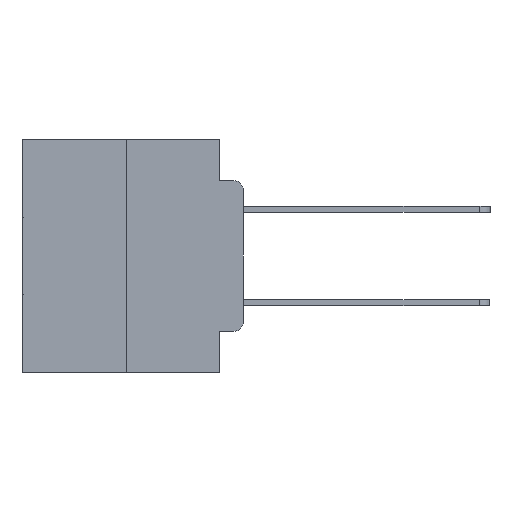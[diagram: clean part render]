
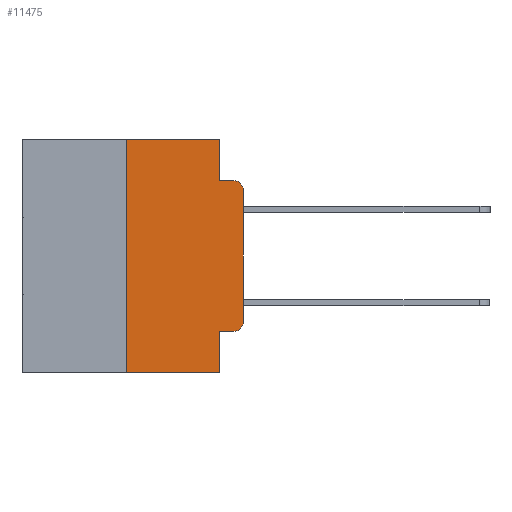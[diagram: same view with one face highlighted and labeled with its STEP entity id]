
A CAD part, left-side view. The second image highlights one B-rep face of the part: STEP entity #11475.
In plain terms, the highlighted planar face has unit normal (-1, 0, 0).
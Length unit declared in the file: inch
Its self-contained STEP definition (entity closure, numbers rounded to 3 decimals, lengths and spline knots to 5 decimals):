
#230 = ORIENTED_EDGE ( 'NONE', *, *, #17750, .T. ) ;
#252 = LINE ( 'NONE', #5214, #23738 ) ;
#612 = ORIENTED_EDGE ( 'NONE', *, *, #15065, .T. ) ;
#625 = EDGE_CURVE ( 'NONE', #12171, #2287, #17639, .T. ) ;
#962 = ORIENTED_EDGE ( 'NONE', *, *, #28681, .F. ) ;
#1080 = VERTEX_POINT ( 'NONE', #4352 ) ;
#1365 = LINE ( 'NONE', #23403, #6791 ) ;
#1390 = FACE_OUTER_BOUND ( 'NONE', #8473, .T. ) ;
#1989 = DIRECTION ( 'NONE',  ( 0., -1., 0. ) ) ;
#2067 = DIRECTION ( 'NONE',  ( -1., 0., 0. ) ) ;
#2287 = VERTEX_POINT ( 'NONE', #5164 ) ;
#2315 = CIRCLE ( 'NONE', #28119, 0.02 ) ;
#3079 = DIRECTION ( 'NONE',  ( -1., 0., 0. ) ) ;
#3886 = ORIENTED_EDGE ( 'NONE', *, *, #11709, .F. ) ;
#4024 = EDGE_CURVE ( 'NONE', #12171, #8507, #252, .T. ) ;
#4352 = CARTESIAN_POINT ( 'NONE',  ( 0., 0.051, 0. ) ) ;
#4429 = CARTESIAN_POINT ( 'NONE',  ( 0., 0.25, 0. ) ) ;
#4977 = LINE ( 'NONE', #8878, #28189 ) ;
#5164 = CARTESIAN_POINT ( 'NONE',  ( 0., 0.051, -0.5 ) ) ;
#5214 = CARTESIAN_POINT ( 'NONE',  ( 0., 0.25, 0. ) ) ;
#5328 = CARTESIAN_POINT ( 'NONE',  ( 0., 0.473, -0.5 ) ) ;
#5348 = CARTESIAN_POINT ( 'NONE',  ( 0., 0., -0.1085 ) ) ;
#5417 = CARTESIAN_POINT ( 'NONE',  ( 0., 0.473, 0. ) ) ;
#5999 = DIRECTION ( 'NONE',  ( 0., -1., 0. ) ) ;
#6517 = EDGE_CURVE ( 'NONE', #9970, #18839, #2315, .T. ) ;
#6551 = VERTEX_POINT ( 'NONE', #18151 ) ;
#6791 = VECTOR ( 'NONE', #10105, 39.37008 ) ;
#6991 = LINE ( 'NONE', #15719, #7715 ) ;
#7275 = VERTEX_POINT ( 'NONE', #16354 ) ;
#7715 = VECTOR ( 'NONE', #1989, 39.37008 ) ;
#7823 = ORIENTED_EDGE ( 'NONE', *, *, #12040, .F. ) ;
#8458 = EDGE_CURVE ( 'NONE', #6551, #18839, #6991, .T. ) ;
#8473 = EDGE_LOOP ( 'NONE', ( #230, #12473, #25096, #962, #7823, #20603, #8550, #3886, #21295, #612 ) ) ;
#8507 = VERTEX_POINT ( 'NONE', #4429 ) ;
#8550 = ORIENTED_EDGE ( 'NONE', *, *, #625, .T. ) ;
#8878 = CARTESIAN_POINT ( 'NONE',  ( 0., 0.473, 0. ) ) ;
#8984 = EDGE_CURVE ( 'NONE', #25645, #19336, #23582, .T. ) ;
#9636 = CIRCLE ( 'NONE', #21478, 0.02 ) ;
#9970 = VERTEX_POINT ( 'NONE', #5348 ) ;
#10105 = DIRECTION ( 'NONE',  ( 0., 0., -1. ) ) ;
#11475 = ADVANCED_FACE ( 'NONE', ( #1390 ), #21213, .F. ) ;
#11626 = VECTOR ( 'NONE', #5999, 39.37008 ) ;
#11639 = VECTOR ( 'NONE', #16133, 39.37008 ) ;
#11709 = EDGE_CURVE ( 'NONE', #25645, #2287, #1365, .T. ) ;
#12040 = EDGE_CURVE ( 'NONE', #8507, #1080, #4977, .T. ) ;
#12086 = DIRECTION ( 'NONE',  ( 0., 0., 1. ) ) ;
#12171 = VERTEX_POINT ( 'NONE', #13817 ) ;
#12231 = CARTESIAN_POINT ( 'NONE',  ( 0., 0.02, -0.0885 ) ) ;
#12473 = ORIENTED_EDGE ( 'NONE', *, *, #6517, .T. ) ;
#13605 = AXIS2_PLACEMENT_3D ( 'NONE', #5417, #27938, #14601 ) ;
#13817 = CARTESIAN_POINT ( 'NONE',  ( 0., 0.25, -0.5 ) ) ;
#14601 = DIRECTION ( 'NONE',  ( 0., 0., -1. ) ) ;
#15065 = EDGE_CURVE ( 'NONE', #19336, #7275, #9636, .T. ) ;
#15082 = CARTESIAN_POINT ( 'NONE',  ( 0., 0.051, -0.4115 ) ) ;
#15719 = CARTESIAN_POINT ( 'NONE',  ( 0., 0.051, -0.0885 ) ) ;
#15800 = CARTESIAN_POINT ( 'NONE',  ( 0., 0.02, -0.1085 ) ) ;
#16133 = DIRECTION ( 'NONE',  ( 0., -1., 0. ) ) ;
#16354 = CARTESIAN_POINT ( 'NONE',  ( 0., 0., -0.3915 ) ) ;
#16526 = CARTESIAN_POINT ( 'NONE',  ( 0., 0.051, 0. ) ) ;
#16618 = LINE ( 'NONE', #17299, #21872 ) ;
#16758 = CARTESIAN_POINT ( 'NONE',  ( 0., 0.02, -0.3915 ) ) ;
#17299 = CARTESIAN_POINT ( 'NONE',  ( 0., 0., 0. ) ) ;
#17639 = LINE ( 'NONE', #5328, #11639 ) ;
#17750 = EDGE_CURVE ( 'NONE', #7275, #9970, #16618, .T. ) ;
#18049 = DIRECTION ( 'NONE',  ( 0., 0., -1. ) ) ;
#18151 = CARTESIAN_POINT ( 'NONE',  ( 0., 0.051, -0.0885 ) ) ;
#18589 = LINE ( 'NONE', #16526, #23822 ) ;
#18788 = DIRECTION ( 'NONE',  ( 0., 0., -1. ) ) ;
#18839 = VERTEX_POINT ( 'NONE', #12231 ) ;
#19013 = DIRECTION ( 'NONE',  ( 0., 0., -1. ) ) ;
#19336 = VERTEX_POINT ( 'NONE', #26618 ) ;
#20603 = ORIENTED_EDGE ( 'NONE', *, *, #4024, .F. ) ;
#21213 = PLANE ( 'NONE',  #13605 ) ;
#21295 = ORIENTED_EDGE ( 'NONE', *, *, #8984, .T. ) ;
#21478 = AXIS2_PLACEMENT_3D ( 'NONE', #16758, #3079, #19013 ) ;
#21872 = VECTOR ( 'NONE', #23953, 39.37008 ) ;
#22409 = DIRECTION ( 'NONE',  ( 0., -1., 0. ) ) ;
#23403 = CARTESIAN_POINT ( 'NONE',  ( 0., 0.051, 0. ) ) ;
#23582 = LINE ( 'NONE', #15082, #11626 ) ;
#23738 = VECTOR ( 'NONE', #12086, 39.37008 ) ;
#23822 = VECTOR ( 'NONE', #18788, 39.37008 ) ;
#23953 = DIRECTION ( 'NONE',  ( 0., 0., 1. ) ) ;
#25096 = ORIENTED_EDGE ( 'NONE', *, *, #8458, .F. ) ;
#25645 = VERTEX_POINT ( 'NONE', #26145 ) ;
#26145 = CARTESIAN_POINT ( 'NONE',  ( 0., 0.051, -0.4115 ) ) ;
#26618 = CARTESIAN_POINT ( 'NONE',  ( 0., 0.02, -0.4115 ) ) ;
#27938 = DIRECTION ( 'NONE',  ( 1., 0., 0. ) ) ;
#28119 = AXIS2_PLACEMENT_3D ( 'NONE', #15800, #2067, #18049 ) ;
#28189 = VECTOR ( 'NONE', #22409, 39.37008 ) ;
#28681 = EDGE_CURVE ( 'NONE', #1080, #6551, #18589, .T. ) ;
